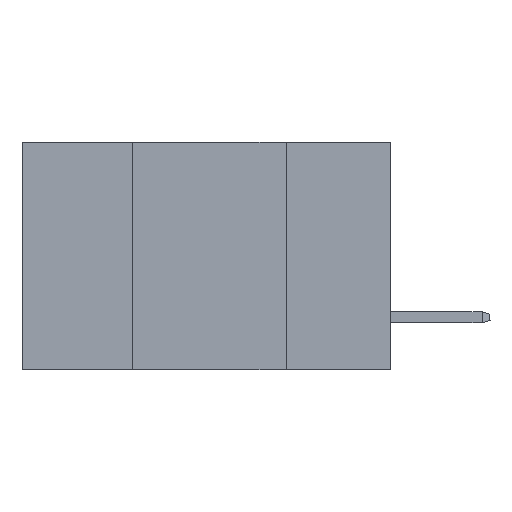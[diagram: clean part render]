
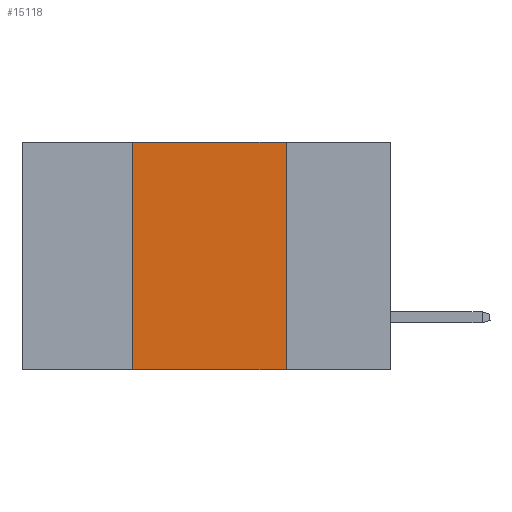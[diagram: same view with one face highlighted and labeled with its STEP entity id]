
A CAD part, left-side view. The second image highlights one B-rep face of the part: STEP entity #15118.
In plain terms, the highlighted planar face has unit normal (-1, 0, 0).
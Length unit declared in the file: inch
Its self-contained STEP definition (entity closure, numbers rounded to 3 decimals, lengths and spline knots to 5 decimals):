
#66 = CARTESIAN_POINT ( 'NONE',  ( 0., 0.17, 0. ) ) ;
#468 = ORIENTED_EDGE ( 'NONE', *, *, #13534, .T. ) ;
#697 = VECTOR ( 'NONE', #6853, 39.37008 ) ;
#1398 = VERTEX_POINT ( 'NONE', #9253 ) ;
#1534 = ORIENTED_EDGE ( 'NONE', *, *, #4433, .F. ) ;
#1578 = VECTOR ( 'NONE', #5416, 39.37008 ) ;
#1778 = LINE ( 'NONE', #66, #1578 ) ;
#1904 = CARTESIAN_POINT ( 'NONE',  ( 0., 0.6, -0.37 ) ) ;
#2444 = DIRECTION ( 'NONE',  ( 0., -1., 0. ) ) ;
#3599 = PLANE ( 'NONE',  #6765 ) ;
#4269 = CARTESIAN_POINT ( 'NONE',  ( 0., 0.42, 0. ) ) ;
#4422 = ORIENTED_EDGE ( 'NONE', *, *, #9275, .F. ) ;
#4433 = EDGE_CURVE ( 'NONE', #1398, #4554, #1778, .T. ) ;
#4554 = VERTEX_POINT ( 'NONE', #11181 ) ;
#4692 = DIRECTION ( 'NONE',  ( 0., -1., 0. ) ) ;
#5054 = EDGE_CURVE ( 'NONE', #14053, #16305, #11335, .T. ) ;
#5105 = CARTESIAN_POINT ( 'NONE',  ( 0., 0.6, 0. ) ) ;
#5190 = LINE ( 'NONE', #5105, #8361 ) ;
#5416 = DIRECTION ( 'NONE',  ( 0., 0., -1. ) ) ;
#6765 = AXIS2_PLACEMENT_3D ( 'NONE', #15683, #8888, #11629 ) ;
#6853 = DIRECTION ( 'NONE',  ( 0., 0., 1. ) ) ;
#7316 = CARTESIAN_POINT ( 'NONE',  ( 0., 0.42, 0. ) ) ;
#8361 = VECTOR ( 'NONE', #2444, 39.37008 ) ;
#8888 = DIRECTION ( 'NONE',  ( 1., 0., 0. ) ) ;
#9253 = CARTESIAN_POINT ( 'NONE',  ( 0., 0.17, 0. ) ) ;
#9275 = EDGE_CURVE ( 'NONE', #16305, #1398, #5190, .T. ) ;
#9834 = EDGE_LOOP ( 'NONE', ( #1534, #4422, #10460, #468 ) ) ;
#10460 = ORIENTED_EDGE ( 'NONE', *, *, #5054, .F. ) ;
#11181 = CARTESIAN_POINT ( 'NONE',  ( 0., 0.17, -0.37 ) ) ;
#11335 = LINE ( 'NONE', #4269, #697 ) ;
#11629 = DIRECTION ( 'NONE',  ( 0., 0., -1. ) ) ;
#13222 = LINE ( 'NONE', #1904, #16386 ) ;
#13534 = EDGE_CURVE ( 'NONE', #14053, #4554, #13222, .T. ) ;
#13601 = FACE_OUTER_BOUND ( 'NONE', #9834, .T. ) ;
#14053 = VERTEX_POINT ( 'NONE', #16392 ) ;
#15118 = ADVANCED_FACE ( 'NONE', ( #13601 ), #3599, .F. ) ;
#15683 = CARTESIAN_POINT ( 'NONE',  ( 0., 0.6, 0. ) ) ;
#16305 = VERTEX_POINT ( 'NONE', #7316 ) ;
#16386 = VECTOR ( 'NONE', #4692, 39.37008 ) ;
#16392 = CARTESIAN_POINT ( 'NONE',  ( 0., 0.42, -0.37 ) ) ;
